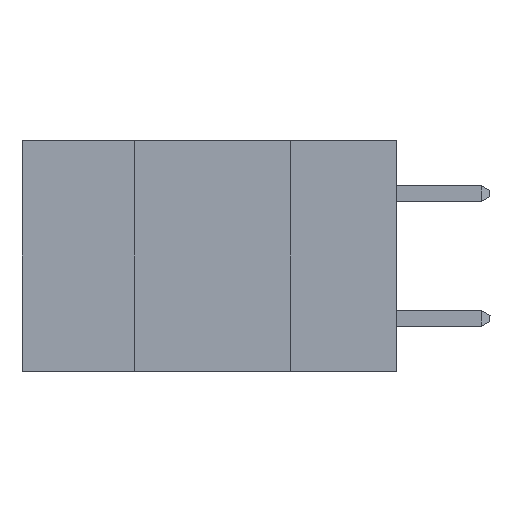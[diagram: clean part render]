
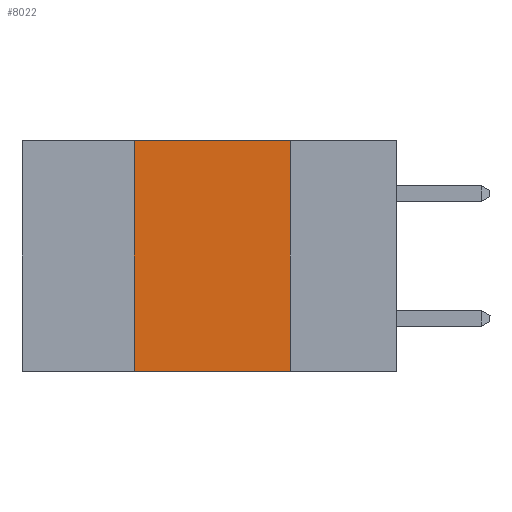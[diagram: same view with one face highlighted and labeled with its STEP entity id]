
A CAD part, left-side view. The second image highlights one B-rep face of the part: STEP entity #8022.
In plain terms, the highlighted planar face has unit normal (-1, 0, 0).
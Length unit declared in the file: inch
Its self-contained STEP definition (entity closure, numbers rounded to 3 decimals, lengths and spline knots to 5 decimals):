
#506 = DIRECTION ( 'NONE',  ( 0., 0., 1. ) ) ;
#1087 = VECTOR ( 'NONE', #9973, 39.37008 ) ;
#1172 = CARTESIAN_POINT ( 'NONE',  ( 0., 0.42, 0. ) ) ;
#1634 = ORIENTED_EDGE ( 'NONE', *, *, #4057, .F. ) ;
#1738 = DIRECTION ( 'NONE',  ( 0., -1., 0. ) ) ;
#1881 = CARTESIAN_POINT ( 'NONE',  ( 0., 0.6, 0. ) ) ;
#3171 = VECTOR ( 'NONE', #17245, 39.37008 ) ;
#3191 = LINE ( 'NONE', #1881, #16549 ) ;
#3431 = VERTEX_POINT ( 'NONE', #18730 ) ;
#3984 = DIRECTION ( 'NONE',  ( 0., 0., -1. ) ) ;
#4057 = EDGE_CURVE ( 'NONE', #3431, #11310, #12535, .T. ) ;
#5200 = FACE_OUTER_BOUND ( 'NONE', #16643, .T. ) ;
#6833 = CARTESIAN_POINT ( 'NONE',  ( 0., 0.6, 0. ) ) ;
#6895 = DIRECTION ( 'NONE',  ( 1., 0., 0. ) ) ;
#7028 = CARTESIAN_POINT ( 'NONE',  ( 0., 0.6, -0.37 ) ) ;
#7033 = VERTEX_POINT ( 'NONE', #17999 ) ;
#7726 = CARTESIAN_POINT ( 'NONE',  ( 0., 0.42, 0. ) ) ;
#8022 = ADVANCED_FACE ( 'NONE', ( #5200 ), #15652, .F. ) ;
#8045 = VERTEX_POINT ( 'NONE', #14557 ) ;
#8158 = VECTOR ( 'NONE', #506, 39.37008 ) ;
#9973 = DIRECTION ( 'NONE',  ( 0., 0., -1. ) ) ;
#11224 = EDGE_CURVE ( 'NONE', #3431, #7033, #11452, .T. ) ;
#11263 = CARTESIAN_POINT ( 'NONE',  ( 0., 0.17, 0. ) ) ;
#11305 = EDGE_CURVE ( 'NONE', #8045, #7033, #16287, .T. ) ;
#11310 = VERTEX_POINT ( 'NONE', #1172 ) ;
#11452 = LINE ( 'NONE', #7028, #3171 ) ;
#12535 = LINE ( 'NONE', #7726, #8158 ) ;
#14557 = CARTESIAN_POINT ( 'NONE',  ( 0., 0.17, 0. ) ) ;
#15652 = PLANE ( 'NONE',  #16255 ) ;
#15655 = ORIENTED_EDGE ( 'NONE', *, *, #11305, .F. ) ;
#15922 = EDGE_CURVE ( 'NONE', #11310, #8045, #3191, .T. ) ;
#16255 = AXIS2_PLACEMENT_3D ( 'NONE', #6833, #6895, #3984 ) ;
#16287 = LINE ( 'NONE', #11263, #1087 ) ;
#16549 = VECTOR ( 'NONE', #1738, 39.37008 ) ;
#16643 = EDGE_LOOP ( 'NONE', ( #15655, #17096, #1634, #18858 ) ) ;
#17096 = ORIENTED_EDGE ( 'NONE', *, *, #15922, .F. ) ;
#17245 = DIRECTION ( 'NONE',  ( 0., -1., 0. ) ) ;
#17999 = CARTESIAN_POINT ( 'NONE',  ( 0., 0.17, -0.37 ) ) ;
#18730 = CARTESIAN_POINT ( 'NONE',  ( 0., 0.42, -0.37 ) ) ;
#18858 = ORIENTED_EDGE ( 'NONE', *, *, #11224, .T. ) ;
